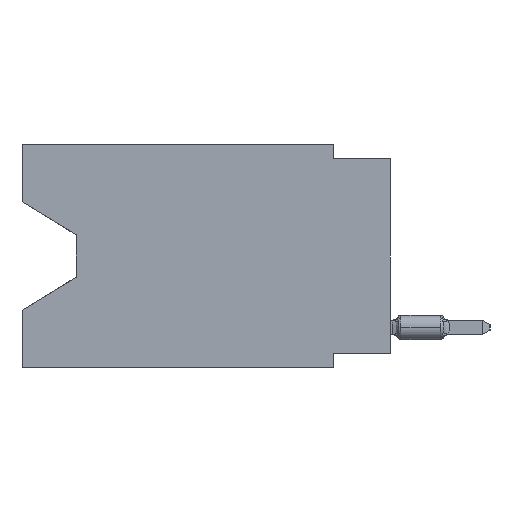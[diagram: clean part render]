
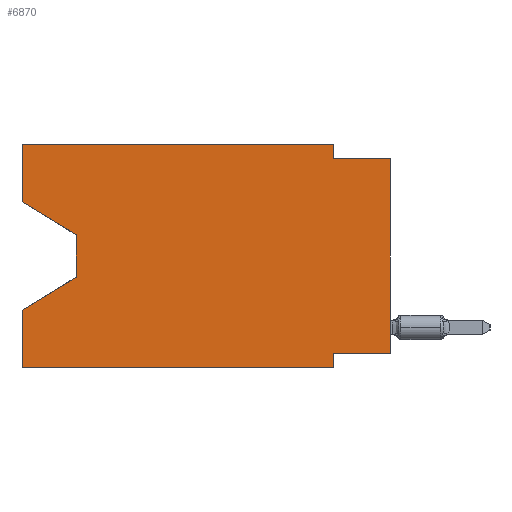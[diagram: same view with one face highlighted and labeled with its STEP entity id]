
A CAD part, left-side view. The second image highlights one B-rep face of the part: STEP entity #6870.
In plain terms, the highlighted planar face has unit normal (-1, 0, 0).
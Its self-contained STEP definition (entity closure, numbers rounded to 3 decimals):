
#448 = CARTESIAN_POINT ( 'NONE',  ( 0., 16.383, -7.36 ) ) ;
#1194 = ORIENTED_EDGE ( 'NONE', *, *, #21916, .T. ) ;
#1815 = CARTESIAN_POINT ( 'NONE',  ( 0., 16.383, 0. ) ) ;
#2632 = CARTESIAN_POINT ( 'NONE',  ( 0., 16.383, -9.906 ) ) ;
#3495 = ORIENTED_EDGE ( 'NONE', *, *, #25574, .F. ) ;
#4414 = VECTOR ( 'NONE', #28624, 1000. ) ;
#4769 = LINE ( 'NONE', #8679, #22260 ) ;
#4827 = CARTESIAN_POINT ( 'NONE',  ( 0., 0., -9.271 ) ) ;
#5288 = CARTESIAN_POINT ( 'NONE',  ( 0., 0., -0.635 ) ) ;
#6695 = EDGE_CURVE ( 'NONE', #19444, #10547, #56418, .T. ) ;
#6870 = ADVANCED_FACE ( 'NONE', ( #55168 ), #10412, .F. ) ;
#7358 = DIRECTION ( 'NONE',  ( 0., -1., 0. ) ) ;
#8573 = DIRECTION ( 'NONE',  ( 0., 0., 1. ) ) ;
#8658 = CARTESIAN_POINT ( 'NONE',  ( 0., 13.97, -4.013 ) ) ;
#8679 = CARTESIAN_POINT ( 'NONE',  ( 0., 2.54, -9.906 ) ) ;
#9000 = ORIENTED_EDGE ( 'NONE', *, *, #26506, .F. ) ;
#9666 = EDGE_CURVE ( 'NONE', #59063, #19444, #18838, .T. ) ;
#9722 = ORIENTED_EDGE ( 'NONE', *, *, #38298, .F. ) ;
#9820 = DIRECTION ( 'NONE',  ( 1., 0., 0. ) ) ;
#9871 = ORIENTED_EDGE ( 'NONE', *, *, #53363, .T. ) ;
#10412 = PLANE ( 'NONE',  #14506 ) ;
#10547 = VERTEX_POINT ( 'NONE', #448 ) ;
#10837 = LINE ( 'NONE', #29152, #45949 ) ;
#12444 = CARTESIAN_POINT ( 'NONE',  ( 0., 0., -0.635 ) ) ;
#12453 = ORIENTED_EDGE ( 'NONE', *, *, #6695, .T. ) ;
#12749 = CARTESIAN_POINT ( 'NONE',  ( 0., 13.97, -4.013 ) ) ;
#12757 = CARTESIAN_POINT ( 'NONE',  ( 0., 2.54, -9.271 ) ) ;
#13151 = CARTESIAN_POINT ( 'NONE',  ( 0., 2.54, -0.635 ) ) ;
#14100 = VERTEX_POINT ( 'NONE', #58700 ) ;
#14506 = AXIS2_PLACEMENT_3D ( 'NONE', #27572, #9820, #23937 ) ;
#14611 = VERTEX_POINT ( 'NONE', #13151 ) ;
#14785 = CARTESIAN_POINT ( 'NONE',  ( 0., 2.54, 0. ) ) ;
#15646 = VECTOR ( 'NONE', #8573, 1000. ) ;
#15753 = EDGE_CURVE ( 'NONE', #26049, #14611, #24971, .T. ) ;
#16477 = DIRECTION ( 'NONE',  ( 0., 0.855, -0.519 ) ) ;
#17301 = LINE ( 'NONE', #2632, #44879 ) ;
#17874 = ORIENTED_EDGE ( 'NONE', *, *, #39735, .T. ) ;
#18631 = LINE ( 'NONE', #4827, #29098 ) ;
#18838 = LINE ( 'NONE', #8658, #42391 ) ;
#19314 = LINE ( 'NONE', #51136, #4414 ) ;
#19444 = VERTEX_POINT ( 'NONE', #49080 ) ;
#19518 = DIRECTION ( 'NONE',  ( 0., 1., 0. ) ) ;
#19655 = VERTEX_POINT ( 'NONE', #12757 ) ;
#20536 = DIRECTION ( 'NONE',  ( 0., -1., 0. ) ) ;
#20798 = CARTESIAN_POINT ( 'NONE',  ( 0., 0., -9.271 ) ) ;
#21869 = VERTEX_POINT ( 'NONE', #20798 ) ;
#21916 = EDGE_CURVE ( 'NONE', #28628, #59063, #36729, .T. ) ;
#22260 = VECTOR ( 'NONE', #36284, 1000. ) ;
#23937 = DIRECTION ( 'NONE',  ( 0., 0., -1. ) ) ;
#24971 = LINE ( 'NONE', #38475, #53009 ) ;
#25194 = VECTOR ( 'NONE', #20536, 1000. ) ;
#25574 = EDGE_CURVE ( 'NONE', #28628, #26616, #50278, .T. ) ;
#25812 = EDGE_CURVE ( 'NONE', #26616, #26049, #43339, .T. ) ;
#26049 = VERTEX_POINT ( 'NONE', #14785 ) ;
#26506 = EDGE_CURVE ( 'NONE', #21869, #19655, #18631, .T. ) ;
#26616 = VERTEX_POINT ( 'NONE', #1815 ) ;
#27572 = CARTESIAN_POINT ( 'NONE',  ( 0., 16.383, 0. ) ) ;
#28028 = ORIENTED_EDGE ( 'NONE', *, *, #9666, .T. ) ;
#28162 = CARTESIAN_POINT ( 'NONE',  ( 0., 2.54, -9.906 ) ) ;
#28624 = DIRECTION ( 'NONE',  ( 0., 0., 1. ) ) ;
#28628 = VERTEX_POINT ( 'NONE', #28850 ) ;
#28850 = CARTESIAN_POINT ( 'NONE',  ( 0., 16.383, -2.546 ) ) ;
#29098 = VECTOR ( 'NONE', #19518, 1000. ) ;
#29152 = CARTESIAN_POINT ( 'NONE',  ( 0., 0., 0. ) ) ;
#29818 = EDGE_CURVE ( 'NONE', #14100, #10547, #19314, .T. ) ;
#30160 = ORIENTED_EDGE ( 'NONE', *, *, #41436, .F. ) ;
#30749 = LINE ( 'NONE', #12444, #39237 ) ;
#32231 = VERTEX_POINT ( 'NONE', #28162 ) ;
#35603 = DIRECTION ( 'NONE',  ( 0., -1., 0. ) ) ;
#36131 = CARTESIAN_POINT ( 'NONE',  ( 0., 16.383, -2.546 ) ) ;
#36284 = DIRECTION ( 'NONE',  ( 0., 0., -1. ) ) ;
#36433 = DIRECTION ( 'NONE',  ( 0., -0.855, -0.519 ) ) ;
#36729 = LINE ( 'NONE', #36131, #41987 ) ;
#38298 = EDGE_CURVE ( 'NONE', #19655, #32231, #4769, .T. ) ;
#38475 = CARTESIAN_POINT ( 'NONE',  ( 0., 2.54, 0. ) ) ;
#38680 = ORIENTED_EDGE ( 'NONE', *, *, #15753, .F. ) ;
#38769 = DIRECTION ( 'NONE',  ( 0., 0., -1. ) ) ;
#39237 = VECTOR ( 'NONE', #7358, 1000. ) ;
#39735 = EDGE_CURVE ( 'NONE', #14100, #32231, #17301, .T. ) ;
#41242 = ORIENTED_EDGE ( 'NONE', *, *, #29818, .F. ) ;
#41436 = EDGE_CURVE ( 'NONE', #14611, #53990, #30749, .T. ) ;
#41987 = VECTOR ( 'NONE', #36433, 1000. ) ;
#42391 = VECTOR ( 'NONE', #55454, 1000. ) ;
#43339 = LINE ( 'NONE', #48429, #25194 ) ;
#44879 = VECTOR ( 'NONE', #35603, 1000. ) ;
#45949 = VECTOR ( 'NONE', #53725, 1000. ) ;
#48429 = CARTESIAN_POINT ( 'NONE',  ( 0., 16.383, 0. ) ) ;
#48576 = CARTESIAN_POINT ( 'NONE',  ( 0., 13.97, -5.893 ) ) ;
#49080 = CARTESIAN_POINT ( 'NONE',  ( 0., 13.97, -5.893 ) ) ;
#49347 = EDGE_LOOP ( 'NONE', ( #1194, #28028, #12453, #41242, #17874, #9722, #9000, #9871, #30160, #38680, #54221, #3495 ) ) ;
#49686 = CARTESIAN_POINT ( 'NONE',  ( 0., 16.383, 0. ) ) ;
#50278 = LINE ( 'NONE', #49686, #15646 ) ;
#51136 = CARTESIAN_POINT ( 'NONE',  ( 0., 16.383, 0. ) ) ;
#51833 = VECTOR ( 'NONE', #16477, 1000. ) ;
#53009 = VECTOR ( 'NONE', #38769, 1000. ) ;
#53363 = EDGE_CURVE ( 'NONE', #21869, #53990, #10837, .T. ) ;
#53725 = DIRECTION ( 'NONE',  ( 0., 0., 1. ) ) ;
#53990 = VERTEX_POINT ( 'NONE', #5288 ) ;
#54221 = ORIENTED_EDGE ( 'NONE', *, *, #25812, .F. ) ;
#55168 = FACE_OUTER_BOUND ( 'NONE', #49347, .T. ) ;
#55454 = DIRECTION ( 'NONE',  ( 0., 0., -1. ) ) ;
#56418 = LINE ( 'NONE', #48576, #51833 ) ;
#58700 = CARTESIAN_POINT ( 'NONE',  ( 0., 16.383, -9.906 ) ) ;
#59063 = VERTEX_POINT ( 'NONE', #12749 ) ;
